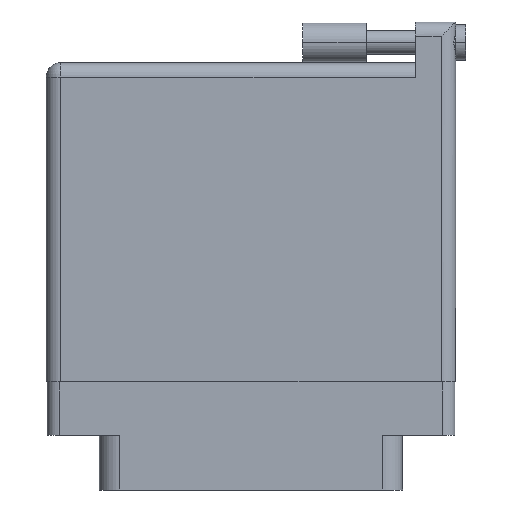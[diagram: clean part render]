
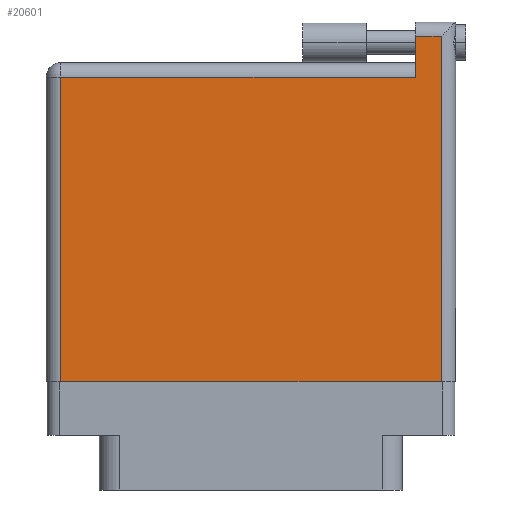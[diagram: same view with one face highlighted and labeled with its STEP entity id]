
A CAD part, front view. The second image highlights one B-rep face of the part: STEP entity #20601.
In plain terms, the highlighted face is planar.
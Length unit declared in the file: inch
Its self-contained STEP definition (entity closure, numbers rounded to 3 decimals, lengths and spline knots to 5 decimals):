
#96 = AXIS2_PLACEMENT_3D ( 'NONE', #22774, #28135, #25213 ) ;
#957 = VECTOR ( 'NONE', #20778, 39.37008 ) ;
#1308 = CARTESIAN_POINT ( 'NONE',  ( 1.811, 1.696, 0. ) ) ;
#1984 = VECTOR ( 'NONE', #25687, 39.37008 ) ;
#3384 = EDGE_CURVE ( 'NONE', #10663, #13914, #4034, .T. ) ;
#4034 = LINE ( 'NONE', #6878, #31668 ) ;
#4228 = CARTESIAN_POINT ( 'NONE',  ( 1.938, 1.696, 0. ) ) ;
#4865 = CARTESIAN_POINT ( 'NONE',  ( 0., 1.696, 0. ) ) ;
#5390 = ORIENTED_EDGE ( 'NONE', *, *, #24699, .T. ) ;
#6878 = CARTESIAN_POINT ( 'NONE',  ( 0., 1.496, 0. ) ) ;
#6903 = CARTESIAN_POINT ( 'NONE',  ( 1.811, 1.496, 0. ) ) ;
#7837 = FACE_OUTER_BOUND ( 'NONE', #31928, .T. ) ;
#8371 = ORIENTED_EDGE ( 'NONE', *, *, #15594, .T. ) ;
#9051 = CARTESIAN_POINT ( 'NONE',  ( 0., 0., 0. ) ) ;
#9125 = LINE ( 'NONE', #28717, #1984 ) ;
#10663 = VERTEX_POINT ( 'NONE', #6903 ) ;
#11649 = EDGE_CURVE ( 'NONE', #21934, #10663, #21102, .T. ) ;
#11876 = CARTESIAN_POINT ( 'NONE',  ( 0.07, 0., 0. ) ) ;
#12410 = ORIENTED_EDGE ( 'NONE', *, *, #27619, .T. ) ;
#13914 = VERTEX_POINT ( 'NONE', #22131 ) ;
#14296 = DIRECTION ( 'NONE',  ( 0., -1., 0. ) ) ;
#14659 = VECTOR ( 'NONE', #14296, 39.37008 ) ;
#15594 = EDGE_CURVE ( 'NONE', #13914, #29152, #16321, .T. ) ;
#16060 = CARTESIAN_POINT ( 'NONE',  ( 1.938, 0., 0. ) ) ;
#16321 = LINE ( 'NONE', #11876, #14659 ) ;
#17254 = VECTOR ( 'NONE', #29542, 39.37008 ) ;
#19881 = PLANE ( 'NONE',  #96 ) ;
#19996 = VECTOR ( 'NONE', #29989, 39.37008 ) ;
#20142 = VERTEX_POINT ( 'NONE', #16060 ) ;
#20601 = ADVANCED_FACE ( 'NONE', ( #7837 ), #19881, .F. ) ;
#20778 = DIRECTION ( 'NONE',  ( 0., -1., 0. ) ) ;
#21102 = LINE ( 'NONE', #31375, #957 ) ;
#21729 = ORIENTED_EDGE ( 'NONE', *, *, #26881, .T. ) ;
#21934 = VERTEX_POINT ( 'NONE', #1308 ) ;
#22131 = CARTESIAN_POINT ( 'NONE',  ( 0.07, 1.496, 0. ) ) ;
#22774 = CARTESIAN_POINT ( 'NONE',  ( 0., 1.566, 0. ) ) ;
#24699 = EDGE_CURVE ( 'NONE', #32592, #21934, #30620, .T. ) ;
#25213 = DIRECTION ( 'NONE',  ( -1., 0., 0. ) ) ;
#25687 = DIRECTION ( 'NONE',  ( 0., 1., 0. ) ) ;
#26881 = EDGE_CURVE ( 'NONE', #20142, #32592, #9125, .T. ) ;
#26952 = ORIENTED_EDGE ( 'NONE', *, *, #11649, .T. ) ;
#27064 = LINE ( 'NONE', #9051, #19996 ) ;
#27619 = EDGE_CURVE ( 'NONE', #29152, #20142, #27064, .T. ) ;
#28135 = DIRECTION ( 'NONE',  ( 0., 0., -1. ) ) ;
#28717 = CARTESIAN_POINT ( 'NONE',  ( 1.938, 1.766, 0. ) ) ;
#28850 = CARTESIAN_POINT ( 'NONE',  ( 0.07, 0., 0. ) ) ;
#29152 = VERTEX_POINT ( 'NONE', #28850 ) ;
#29542 = DIRECTION ( 'NONE',  ( -1., 0., 0. ) ) ;
#29804 = ORIENTED_EDGE ( 'NONE', *, *, #3384, .T. ) ;
#29989 = DIRECTION ( 'NONE',  ( 1., 0., 0. ) ) ;
#30620 = LINE ( 'NONE', #4865, #17254 ) ;
#30976 = DIRECTION ( 'NONE',  ( -1., 0., 0. ) ) ;
#31375 = CARTESIAN_POINT ( 'NONE',  ( 1.811, 1.766, 0. ) ) ;
#31668 = VECTOR ( 'NONE', #30976, 39.37008 ) ;
#31928 = EDGE_LOOP ( 'NONE', ( #12410, #21729, #5390, #26952, #29804, #8371 ) ) ;
#32592 = VERTEX_POINT ( 'NONE', #4228 ) ;
